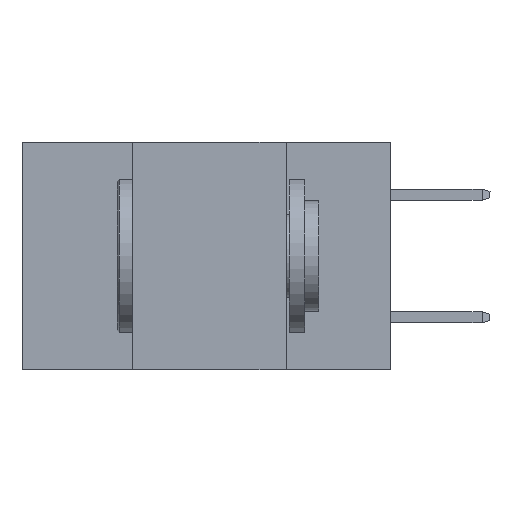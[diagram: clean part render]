
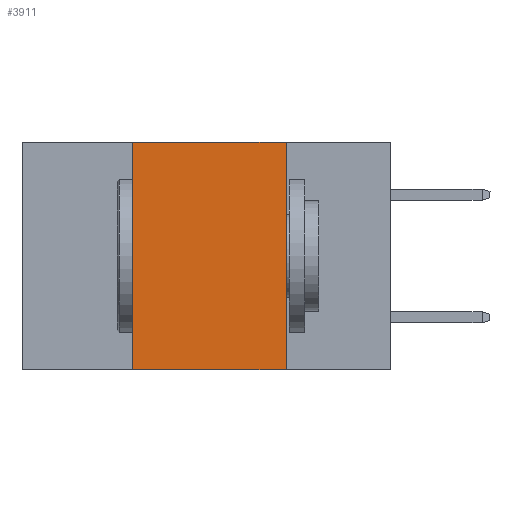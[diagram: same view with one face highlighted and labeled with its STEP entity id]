
A CAD part, left-side view. The second image highlights one B-rep face of the part: STEP entity #3911.
In plain terms, the highlighted planar face has unit normal (-1, 0, 0).
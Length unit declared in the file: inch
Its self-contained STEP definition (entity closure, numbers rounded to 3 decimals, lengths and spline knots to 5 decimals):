
#126 = CARTESIAN_POINT ( 'NONE',  ( 0., 0.17, 0. ) ) ;
#319 = EDGE_CURVE ( 'NONE', #2546, #12128, #11784, .T. ) ;
#1826 = DIRECTION ( 'NONE',  ( 0., -1., 0. ) ) ;
#1836 = CARTESIAN_POINT ( 'NONE',  ( 0., 0.17, -0.37 ) ) ;
#1953 = EDGE_CURVE ( 'NONE', #2546, #13460, #6394, .T. ) ;
#1961 = ORIENTED_EDGE ( 'NONE', *, *, #319, .F. ) ;
#2239 = CARTESIAN_POINT ( 'NONE',  ( 0., 0.42, 0. ) ) ;
#2546 = VERTEX_POINT ( 'NONE', #3118 ) ;
#2661 = CARTESIAN_POINT ( 'NONE',  ( 0., 0.42, 0. ) ) ;
#2950 = DIRECTION ( 'NONE',  ( 0., 0., -1. ) ) ;
#2964 = DIRECTION ( 'NONE',  ( 1., 0., 0. ) ) ;
#3000 = PLANE ( 'NONE',  #5846 ) ;
#3118 = CARTESIAN_POINT ( 'NONE',  ( 0., 0.42, -0.37 ) ) ;
#3121 = VECTOR ( 'NONE', #7699, 39.37008 ) ;
#3122 = CARTESIAN_POINT ( 'NONE',  ( 0., 0.6, 0. ) ) ;
#3520 = VECTOR ( 'NONE', #12765, 39.37008 ) ;
#3633 = VERTEX_POINT ( 'NONE', #10242 ) ;
#3911 = ADVANCED_FACE ( 'NONE', ( #3930 ), #3000, .F. ) ;
#3930 = FACE_OUTER_BOUND ( 'NONE', #11604, .T. ) ;
#5481 = LINE ( 'NONE', #13823, #13990 ) ;
#5846 = AXIS2_PLACEMENT_3D ( 'NONE', #3122, #2964, #2950 ) ;
#6211 = EDGE_CURVE ( 'NONE', #3633, #13460, #6445, .T. ) ;
#6394 = LINE ( 'NONE', #12222, #11758 ) ;
#6445 = LINE ( 'NONE', #126, #3520 ) ;
#7699 = DIRECTION ( 'NONE',  ( 0., 0., 1. ) ) ;
#10242 = CARTESIAN_POINT ( 'NONE',  ( 0., 0.17, 0. ) ) ;
#10613 = ORIENTED_EDGE ( 'NONE', *, *, #6211, .F. ) ;
#10670 = ORIENTED_EDGE ( 'NONE', *, *, #1953, .T. ) ;
#11604 = EDGE_LOOP ( 'NONE', ( #10613, #12870, #1961, #10670 ) ) ;
#11758 = VECTOR ( 'NONE', #12330, 39.37008 ) ;
#11784 = LINE ( 'NONE', #2661, #3121 ) ;
#11948 = EDGE_CURVE ( 'NONE', #12128, #3633, #5481, .T. ) ;
#12128 = VERTEX_POINT ( 'NONE', #2239 ) ;
#12222 = CARTESIAN_POINT ( 'NONE',  ( 0., 0.6, -0.37 ) ) ;
#12330 = DIRECTION ( 'NONE',  ( 0., -1., 0. ) ) ;
#12765 = DIRECTION ( 'NONE',  ( 0., 0., -1. ) ) ;
#12870 = ORIENTED_EDGE ( 'NONE', *, *, #11948, .F. ) ;
#13460 = VERTEX_POINT ( 'NONE', #1836 ) ;
#13823 = CARTESIAN_POINT ( 'NONE',  ( 0., 0.6, 0. ) ) ;
#13990 = VECTOR ( 'NONE', #1826, 39.37008 ) ;
